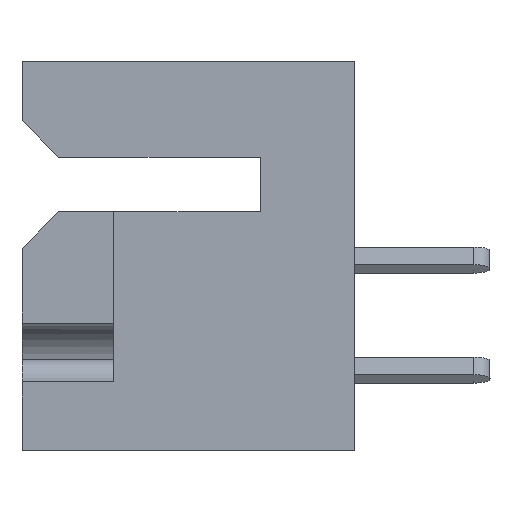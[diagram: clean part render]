
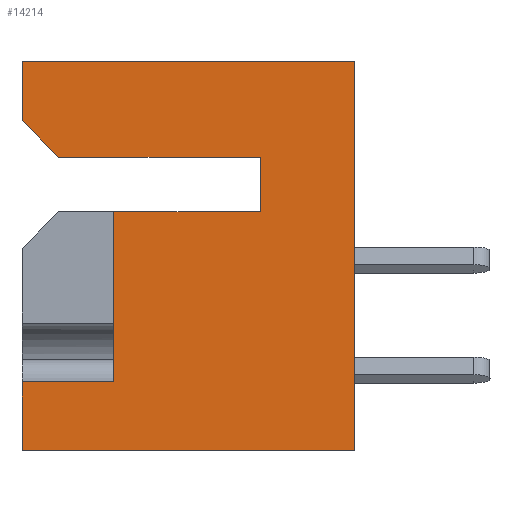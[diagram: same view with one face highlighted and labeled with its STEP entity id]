
A CAD part, left-side view. The second image highlights one B-rep face of the part: STEP entity #14214.
In plain terms, the highlighted planar face has unit normal (-1, 0, 0).
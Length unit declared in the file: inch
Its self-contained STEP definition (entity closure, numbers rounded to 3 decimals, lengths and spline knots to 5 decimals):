
#244 = CARTESIAN_POINT ( 'NONE',  ( 0., 0.328, -0.437 ) ) ;
#789 = DIRECTION ( 'NONE',  ( 0., -1., 0. ) ) ;
#893 = CARTESIAN_POINT ( 'NONE',  ( 0., 0.128, -0.205 ) ) ;
#1155 = VERTEX_POINT ( 'NONE', #893 ) ;
#1339 = LINE ( 'NONE', #12243, #6561 ) ;
#1630 = LINE ( 'NONE', #25726, #21320 ) ;
#2748 = VERTEX_POINT ( 'NONE', #8438 ) ;
#2927 = EDGE_CURVE ( 'NONE', #19340, #18676, #9842, .T. ) ;
#3116 = ORIENTED_EDGE ( 'NONE', *, *, #23522, .T. ) ;
#3847 = ORIENTED_EDGE ( 'NONE', *, *, #7590, .T. ) ;
#4100 = ORIENTED_EDGE ( 'NONE', *, *, #28339, .F. ) ;
#4590 = DIRECTION ( 'NONE',  ( 1., 0., 0. ) ) ;
#5455 = ORIENTED_EDGE ( 'NONE', *, *, #2927, .T. ) ;
#5584 = ORIENTED_EDGE ( 'NONE', *, *, #8386, .T. ) ;
#6561 = VECTOR ( 'NONE', #7880, 39.37008 ) ;
#7250 = VERTEX_POINT ( 'NONE', #10775 ) ;
#7506 = VERTEX_POINT ( 'NONE', #20574 ) ;
#7590 = EDGE_CURVE ( 'NONE', #18676, #7250, #13928, .T. ) ;
#7737 = ORIENTED_EDGE ( 'NONE', *, *, #22961, .F. ) ;
#7880 = DIRECTION ( 'NONE',  ( 0., 1., 0. ) ) ;
#7882 = VERTEX_POINT ( 'NONE', #8682 ) ;
#8179 = EDGE_CURVE ( 'NONE', #25563, #16967, #24573, .T. ) ;
#8386 = EDGE_CURVE ( 'NONE', #1155, #2748, #27293, .T. ) ;
#8438 = CARTESIAN_POINT ( 'NONE',  ( 0., 0.328, -0.205 ) ) ;
#8600 = CARTESIAN_POINT ( 'NONE',  ( 0., 0.128, -0.131 ) ) ;
#8682 = CARTESIAN_POINT ( 'NONE',  ( 0., 0.128, -0.131 ) ) ;
#8985 = LINE ( 'NONE', #22080, #24855 ) ;
#9834 = FACE_OUTER_BOUND ( 'NONE', #14376, .T. ) ;
#9842 = LINE ( 'NONE', #22770, #27750 ) ;
#10099 = VECTOR ( 'NONE', #27181, 39.37008 ) ;
#10648 = CARTESIAN_POINT ( 'NONE',  ( 0., 0.453, -0.081 ) ) ;
#10711 = EDGE_CURVE ( 'NONE', #1155, #7882, #24177, .T. ) ;
#10775 = CARTESIAN_POINT ( 'NONE',  ( 0., 0., 0. ) ) ;
#11927 = CARTESIAN_POINT ( 'NONE',  ( 0., 0.453, -0.531 ) ) ;
#12243 = CARTESIAN_POINT ( 'NONE',  ( 0., 0.328, -0.437 ) ) ;
#12507 = VECTOR ( 'NONE', #15059, 39.37008 ) ;
#12603 = VERTEX_POINT ( 'NONE', #12815 ) ;
#12745 = ORIENTED_EDGE ( 'NONE', *, *, #23867, .T. ) ;
#12815 = CARTESIAN_POINT ( 'NONE',  ( 0., 0.403, -0.131 ) ) ;
#13096 = CARTESIAN_POINT ( 'NONE',  ( 0., 0.403, -0.131 ) ) ;
#13158 = CARTESIAN_POINT ( 'NONE',  ( 0., 0.453, 0. ) ) ;
#13928 = LINE ( 'NONE', #16440, #10099 ) ;
#14214 = ADVANCED_FACE ( 'NONE', ( #9834 ), #28520, .F. ) ;
#14376 = EDGE_LOOP ( 'NONE', ( #3116, #24447, #5455, #3847, #19989, #28109, #12745, #4100, #27907, #5584, #7737 ) ) ;
#14501 = DIRECTION ( 'NONE',  ( 0., 1., 0. ) ) ;
#14889 = CARTESIAN_POINT ( 'NONE',  ( 0., 0.128, -0.131 ) ) ;
#15059 = DIRECTION ( 'NONE',  ( 0., 0., 1. ) ) ;
#15753 = DIRECTION ( 'NONE',  ( 0., 0., 1. ) ) ;
#16045 = VECTOR ( 'NONE', #14501, 39.37008 ) ;
#16440 = CARTESIAN_POINT ( 'NONE',  ( 0., 0., 0. ) ) ;
#16639 = AXIS2_PLACEMENT_3D ( 'NONE', #22108, #4590, #26626 ) ;
#16967 = VERTEX_POINT ( 'NONE', #23287 ) ;
#18676 = VERTEX_POINT ( 'NONE', #27099 ) ;
#19340 = VERTEX_POINT ( 'NONE', #11927 ) ;
#19989 = ORIENTED_EDGE ( 'NONE', *, *, #26707, .F. ) ;
#20073 = VECTOR ( 'NONE', #24039, 39.37008 ) ;
#20574 = CARTESIAN_POINT ( 'NONE',  ( 0., 0.453, -0.437 ) ) ;
#21320 = VECTOR ( 'NONE', #23451, 39.37008 ) ;
#21359 = VECTOR ( 'NONE', #24278, 39.37008 ) ;
#22080 = CARTESIAN_POINT ( 'NONE',  ( 0., 0.328, -0.205 ) ) ;
#22108 = CARTESIAN_POINT ( 'NONE',  ( 0., 0.453, 0. ) ) ;
#22411 = LINE ( 'NONE', #13158, #20073 ) ;
#22770 = CARTESIAN_POINT ( 'NONE',  ( 0., 0.453, -0.531 ) ) ;
#22772 = VECTOR ( 'NONE', #26237, 39.37008 ) ;
#22961 = EDGE_CURVE ( 'NONE', #23262, #2748, #8985, .T. ) ;
#23262 = VERTEX_POINT ( 'NONE', #244 ) ;
#23287 = CARTESIAN_POINT ( 'NONE',  ( 0., 0.453, 0. ) ) ;
#23451 = DIRECTION ( 'NONE',  ( 0., -1., 0. ) ) ;
#23492 = LINE ( 'NONE', #13096, #21359 ) ;
#23522 = EDGE_CURVE ( 'NONE', #23262, #7506, #1339, .T. ) ;
#23867 = EDGE_CURVE ( 'NONE', #25563, #12603, #23492, .T. ) ;
#24039 = DIRECTION ( 'NONE',  ( 0., 0., 1. ) ) ;
#24062 = DIRECTION ( 'NONE',  ( 0., 1., 0. ) ) ;
#24177 = LINE ( 'NONE', #8600, #22772 ) ;
#24278 = DIRECTION ( 'NONE',  ( 0., -0.707, -0.707 ) ) ;
#24303 = LINE ( 'NONE', #14889, #16045 ) ;
#24387 = EDGE_CURVE ( 'NONE', #19340, #7506, #22411, .T. ) ;
#24447 = ORIENTED_EDGE ( 'NONE', *, *, #24387, .F. ) ;
#24573 = LINE ( 'NONE', #26291, #12507 ) ;
#24855 = VECTOR ( 'NONE', #15753, 39.37008 ) ;
#25563 = VERTEX_POINT ( 'NONE', #10648 ) ;
#25726 = CARTESIAN_POINT ( 'NONE',  ( 0., 0.453, 0. ) ) ;
#26055 = CARTESIAN_POINT ( 'NONE',  ( 0., 0.128, -0.205 ) ) ;
#26237 = DIRECTION ( 'NONE',  ( 0., 0., 1. ) ) ;
#26249 = VECTOR ( 'NONE', #24062, 39.37008 ) ;
#26291 = CARTESIAN_POINT ( 'NONE',  ( 0., 0.453, 0. ) ) ;
#26626 = DIRECTION ( 'NONE',  ( 0., 0., -1. ) ) ;
#26707 = EDGE_CURVE ( 'NONE', #16967, #7250, #1630, .T. ) ;
#27099 = CARTESIAN_POINT ( 'NONE',  ( 0., 0., -0.531 ) ) ;
#27181 = DIRECTION ( 'NONE',  ( 0., 0., 1. ) ) ;
#27293 = LINE ( 'NONE', #26055, #26249 ) ;
#27750 = VECTOR ( 'NONE', #789, 39.37008 ) ;
#27907 = ORIENTED_EDGE ( 'NONE', *, *, #10711, .F. ) ;
#28109 = ORIENTED_EDGE ( 'NONE', *, *, #8179, .F. ) ;
#28339 = EDGE_CURVE ( 'NONE', #7882, #12603, #24303, .T. ) ;
#28520 = PLANE ( 'NONE',  #16639 ) ;
